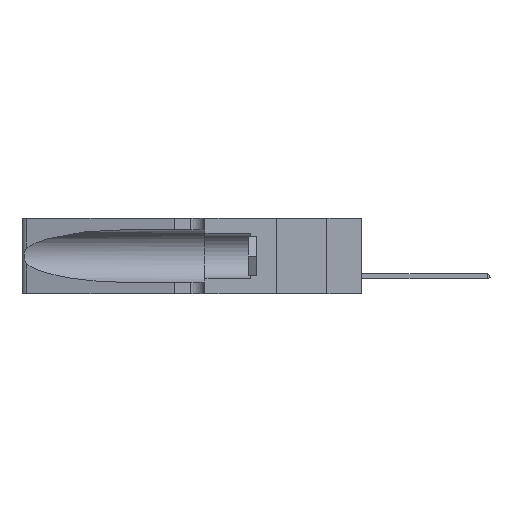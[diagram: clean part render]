
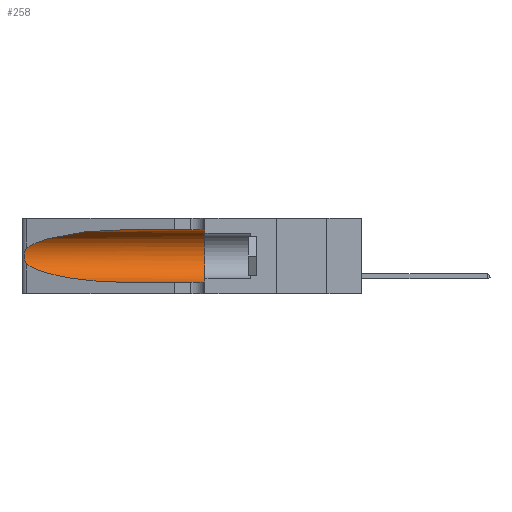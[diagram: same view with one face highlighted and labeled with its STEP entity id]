
A CAD part, left-side view. The second image highlights one B-rep face of the part: STEP entity #258.
In plain terms, the highlighted cylindrical face has radius 3.308 mm (diameter 6.617 mm), a partial arc.
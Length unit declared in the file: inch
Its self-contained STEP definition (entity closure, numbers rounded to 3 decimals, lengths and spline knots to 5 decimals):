
#141 = LINE ( 'NONE', #18341, #1101 ) ;
#222 = ORIENTED_EDGE ( 'NONE', *, *, #11982, .T. ) ;
#258 = ADVANCED_FACE ( 'NONE', ( #16855 ), #7669, .F. ) ;
#1039 = CARTESIAN_POINT ( 'NONE',  ( 0.25639, 1.23184, 0.21858 ) ) ;
#1101 = VECTOR ( 'NONE', #23850, 39.37008 ) ;
#1161 = VECTOR ( 'NONE', #19101, 39.37008 ) ;
#1575 = EDGE_CURVE ( 'NONE', #5293, #16569, #4560, .T. ) ;
#1729 = CARTESIAN_POINT ( 'NONE',  ( 0.18966, 0.96281, 0.05475 ) ) ;
#2103 = DIRECTION ( 'NONE',  ( 0., -1., 0. ) ) ;
#2311 = AXIS2_PLACEMENT_3D ( 'NONE', #11690, #2103, #7739 ) ;
#2445 = CARTESIAN_POINT ( 'NONE',  ( 0.1305, 0.35, 0.05475 ) ) ;
#2637 = AXIS2_PLACEMENT_3D ( 'NONE', #24787, #11095, #21100 ) ;
#2810 = CARTESIAN_POINT ( 'NONE',  ( 0.26075, 1.23896, 0.19203 ) ) ;
#2975 = CARTESIAN_POINT ( 'NONE',  ( 0.25639, 1.23186, 0.15144 ) ) ;
#3052 = ORIENTED_EDGE ( 'NONE', *, *, #7985, .T. ) ;
#3155 = CARTESIAN_POINT ( 'NONE',  ( 0.25487, 1.22718, 0.22369 ) ) ;
#3162 = CARTESIAN_POINT ( 'NONE',  ( 0.2373, 1.15595, 0.28018 ) ) ;
#3710 =( BOUNDED_CURVE ( )  B_SPLINE_CURVE ( 3, ( #21050, #17088, #1729, #15392 ),
 .UNSPECIFIED., .F., .F. ) 
 B_SPLINE_CURVE_WITH_KNOTS ( ( 4, 4 ),
 ( 3.44316, 4.71239 ),
 .UNSPECIFIED. ) 
 CURVE ( )  GEOMETRIC_REPRESENTATION_ITEM ( )  RATIONAL_B_SPLINE_CURVE ( ( 1., 0.87, 0.87, 1. ) ) 
 REPRESENTATION_ITEM ( '' )  );
#4560 = CIRCLE ( 'NONE', #2637, 0.13025 ) ;
#4788 = CARTESIAN_POINT ( 'NONE',  ( 0.26075, 1.23896, 0.178 ) ) ;
#4900 = EDGE_CURVE ( 'NONE', #8474, #12242, #24170, .T. ) ;
#5039 = CARTESIAN_POINT ( 'NONE',  ( 0.25555, 1.22993, 0.14849 ) ) ;
#5293 = VERTEX_POINT ( 'NONE', #13628 ) ;
#6308 = LINE ( 'NONE', #23142, #1161 ) ;
#6621 = CARTESIAN_POINT ( 'NONE',  ( 0.25487, 1.22718, 0.22369 ) ) ;
#6991 = CARTESIAN_POINT ( 'NONE',  ( 0.26017, 1.23833, 0.17102 ) ) ;
#7669 = CYLINDRICAL_SURFACE ( 'NONE', #2311, 0.13025 ) ;
#7739 = DIRECTION ( 'NONE',  ( 0., 0., -1. ) ) ;
#7985 = EDGE_CURVE ( 'NONE', #11733, #24968, #3710, .T. ) ;
#8474 = VERTEX_POINT ( 'NONE', #21096 ) ;
#9001 = CARTESIAN_POINT ( 'NONE',  ( 0.1305, 0.72297, 0.31525 ) ) ;
#9077 = CARTESIAN_POINT ( 'NONE',  ( 0.25789, 1.23486, 0.15765 ) ) ;
#10950 = CARTESIAN_POINT ( 'NONE',  ( 0.25487, 1.22718, 0.14631 ) ) ;
#11095 = DIRECTION ( 'NONE',  ( 0., 1., 0. ) ) ;
#11690 = CARTESIAN_POINT ( 'NONE',  ( 0.1305, 1.61858, 0.185 ) ) ;
#11733 = VERTEX_POINT ( 'NONE', #19935 ) ;
#11842 = EDGE_LOOP ( 'NONE', ( #23116, #222, #3052, #17526, #17517, #14013 ) ) ;
#11982 = EDGE_CURVE ( 'NONE', #12242, #11733, #15143, .T. ) ;
#12242 = VERTEX_POINT ( 'NONE', #6621 ) ;
#13628 = CARTESIAN_POINT ( 'NONE',  ( 0.1305, 0.35, 0.31525 ) ) ;
#14013 = ORIENTED_EDGE ( 'NONE', *, *, #21294, .F. ) ;
#14704 = CARTESIAN_POINT ( 'NONE',  ( 0.18966, 0.96281, 0.31525 ) ) ;
#15143 = B_SPLINE_CURVE_WITH_KNOTS ( 'NONE', 3,
 ( #3155, #16667, #1039, #16836, #22697, #24635, #2810, #4788, #6991, #22451, #9077, #2975, #5039, #10950 ),
 .UNSPECIFIED., .F., .F.,
 ( 4, 2, 2, 2, 2, 2, 4 ),
 ( 0., 0.00027, 0.00053, 0.00107, 0.0016, 0.00187, 0.00214 ),
 .UNSPECIFIED. ) ;
#15335 = EDGE_CURVE ( 'NONE', #24968, #16569, #6308, .T. ) ;
#15392 = CARTESIAN_POINT ( 'NONE',  ( 0.1305, 0.72297, 0.05475 ) ) ;
#16569 = VERTEX_POINT ( 'NONE', #2445 ) ;
#16667 = CARTESIAN_POINT ( 'NONE',  ( 0.25555, 1.22994, 0.2215 ) ) ;
#16836 = CARTESIAN_POINT ( 'NONE',  ( 0.25787, 1.23484, 0.2124 ) ) ;
#16855 = FACE_OUTER_BOUND ( 'NONE', #11842, .T. ) ;
#17088 = CARTESIAN_POINT ( 'NONE',  ( 0.2373, 1.15595, 0.08982 ) ) ;
#17517 = ORIENTED_EDGE ( 'NONE', *, *, #1575, .F. ) ;
#17526 = ORIENTED_EDGE ( 'NONE', *, *, #15335, .T. ) ;
#18341 = CARTESIAN_POINT ( 'NONE',  ( 0.1305, 1.61858, 0.31525 ) ) ;
#18545 = CARTESIAN_POINT ( 'NONE',  ( 0.1305, 0.72297, 0.05475 ) ) ;
#19101 = DIRECTION ( 'NONE',  ( 0., -1., 0. ) ) ;
#19935 = CARTESIAN_POINT ( 'NONE',  ( 0.25487, 1.22718, 0.14631 ) ) ;
#21050 = CARTESIAN_POINT ( 'NONE',  ( 0.25487, 1.22718, 0.14631 ) ) ;
#21096 = CARTESIAN_POINT ( 'NONE',  ( 0.1305, 0.72297, 0.31525 ) ) ;
#21100 = DIRECTION ( 'NONE',  ( 0., 0., 1. ) ) ;
#21294 = EDGE_CURVE ( 'NONE', #8474, #5293, #141, .T. ) ;
#22451 = CARTESIAN_POINT ( 'NONE',  ( 0.25856, 1.23593, 0.16098 ) ) ;
#22697 = CARTESIAN_POINT ( 'NONE',  ( 0.25854, 1.2359, 0.20912 ) ) ;
#23116 = ORIENTED_EDGE ( 'NONE', *, *, #4900, .T. ) ;
#23142 = CARTESIAN_POINT ( 'NONE',  ( 0.1305, 1.61858, 0.05475 ) ) ;
#23850 = DIRECTION ( 'NONE',  ( 0., -1., 0. ) ) ;
#24170 =( BOUNDED_CURVE ( )  B_SPLINE_CURVE ( 3, ( #9001, #14704, #3162, #24481 ),
 .UNSPECIFIED., .F., .T. ) 
 B_SPLINE_CURVE_WITH_KNOTS ( ( 4, 4 ),
 ( 1.5708, 2.84003 ),
 .UNSPECIFIED. ) 
 CURVE ( )  GEOMETRIC_REPRESENTATION_ITEM ( )  RATIONAL_B_SPLINE_CURVE ( ( 1., 0.87, 0.87, 1. ) ) 
 REPRESENTATION_ITEM ( '' )  );
#24481 = CARTESIAN_POINT ( 'NONE',  ( 0.25487, 1.22718, 0.22369 ) ) ;
#24635 = CARTESIAN_POINT ( 'NONE',  ( 0.26018, 1.23835, 0.19895 ) ) ;
#24787 = CARTESIAN_POINT ( 'NONE',  ( 0.1305, 0.35, 0.185 ) ) ;
#24968 = VERTEX_POINT ( 'NONE', #18545 ) ;
